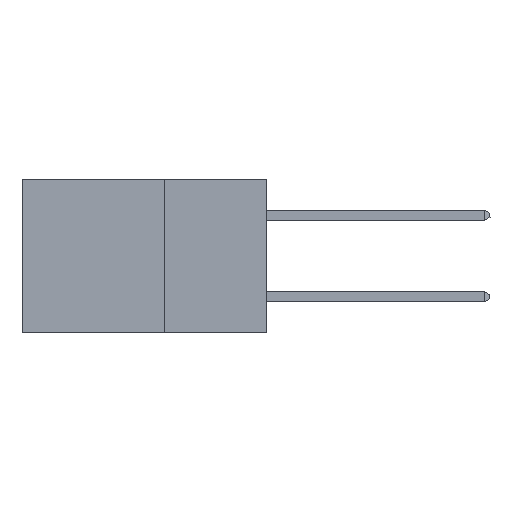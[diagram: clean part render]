
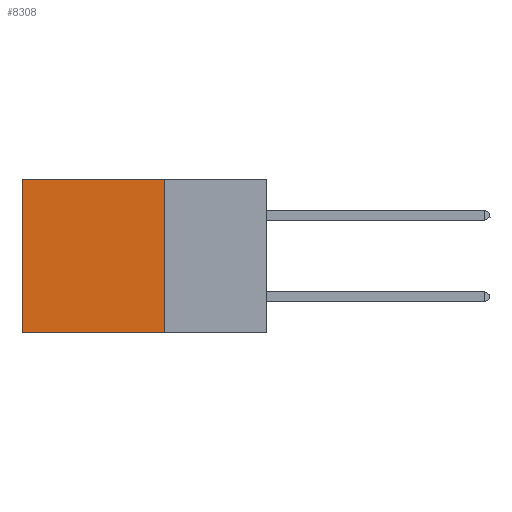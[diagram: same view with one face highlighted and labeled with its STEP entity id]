
A CAD part, left-side view. The second image highlights one B-rep face of the part: STEP entity #8308.
In plain terms, the highlighted planar face has unit normal (-1, 0, 0).
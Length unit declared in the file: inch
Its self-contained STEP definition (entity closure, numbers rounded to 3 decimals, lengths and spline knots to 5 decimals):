
#230 = CARTESIAN_POINT ( 'NONE',  ( 0.2875, 0.25, 0. ) ) ;
#572 = VECTOR ( 'NONE', #4852, 39.37008 ) ;
#652 = FACE_OUTER_BOUND ( 'NONE', #8965, .T. ) ;
#860 = DIRECTION ( 'NONE',  ( 1., 0., 0. ) ) ;
#892 = CARTESIAN_POINT ( 'NONE',  ( 0.2875, 0.25, -0.375 ) ) ;
#1094 = CARTESIAN_POINT ( 'NONE',  ( 0.2875, 0.25, -0.375 ) ) ;
#1687 = CARTESIAN_POINT ( 'NONE',  ( 0.2875, 0.25, -0.375 ) ) ;
#1760 = LINE ( 'NONE', #1687, #572 ) ;
#2091 = LINE ( 'NONE', #1094, #9602 ) ;
#2361 = VERTEX_POINT ( 'NONE', #6929 ) ;
#2454 = ORIENTED_EDGE ( 'NONE', *, *, #3231, .F. ) ;
#2542 = VECTOR ( 'NONE', #7856, 39.37008 ) ;
#2552 = CARTESIAN_POINT ( 'NONE',  ( 0.2875, 0.6, 0. ) ) ;
#2769 = LINE ( 'NONE', #7120, #2542 ) ;
#3036 = ORIENTED_EDGE ( 'NONE', *, *, #4717, .T. ) ;
#3077 = DIRECTION ( 'NONE',  ( 0., 0., -1. ) ) ;
#3231 = EDGE_CURVE ( 'NONE', #8470, #6842, #1760, .T. ) ;
#3693 = CARTESIAN_POINT ( 'NONE',  ( 0.2875, 0.25, 0. ) ) ;
#3842 = CARTESIAN_POINT ( 'NONE',  ( 0.2875, 0.25, -0.375 ) ) ;
#4704 = DIRECTION ( 'NONE',  ( 0., 1., 0. ) ) ;
#4717 = EDGE_CURVE ( 'NONE', #8470, #5059, #5951, .T. ) ;
#4852 = DIRECTION ( 'NONE',  ( 0., 0., -1. ) ) ;
#5059 = VERTEX_POINT ( 'NONE', #2552 ) ;
#5246 = EDGE_CURVE ( 'NONE', #5059, #2361, #2769, .T. ) ;
#5303 = PLANE ( 'NONE',  #7534 ) ;
#5607 = ORIENTED_EDGE ( 'NONE', *, *, #5246, .T. ) ;
#5868 = DIRECTION ( 'NONE',  ( 0., 1., 0. ) ) ;
#5951 = LINE ( 'NONE', #3693, #9020 ) ;
#6278 = EDGE_CURVE ( 'NONE', #6842, #2361, #2091, .T. ) ;
#6333 = ORIENTED_EDGE ( 'NONE', *, *, #6278, .F. ) ;
#6842 = VERTEX_POINT ( 'NONE', #3842 ) ;
#6929 = CARTESIAN_POINT ( 'NONE',  ( 0.2875, 0.6, -0.375 ) ) ;
#7120 = CARTESIAN_POINT ( 'NONE',  ( 0.2875, 0.6, -0.375 ) ) ;
#7534 = AXIS2_PLACEMENT_3D ( 'NONE', #892, #860, #3077 ) ;
#7856 = DIRECTION ( 'NONE',  ( 0., 0., -1. ) ) ;
#8308 = ADVANCED_FACE ( 'NONE', ( #652 ), #5303, .F. ) ;
#8470 = VERTEX_POINT ( 'NONE', #230 ) ;
#8965 = EDGE_LOOP ( 'NONE', ( #5607, #6333, #2454, #3036 ) ) ;
#9020 = VECTOR ( 'NONE', #5868, 39.37008 ) ;
#9602 = VECTOR ( 'NONE', #4704, 39.37008 ) ;
